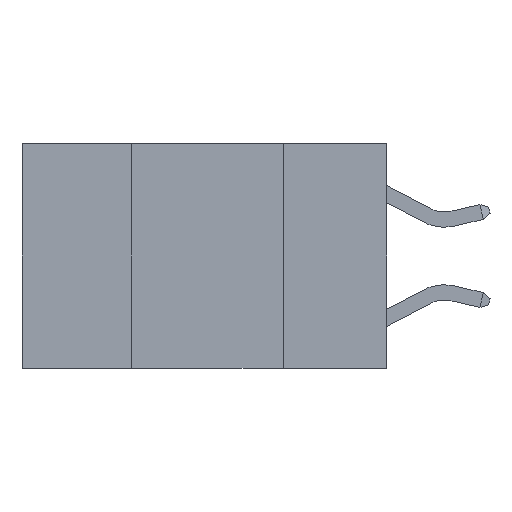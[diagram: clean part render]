
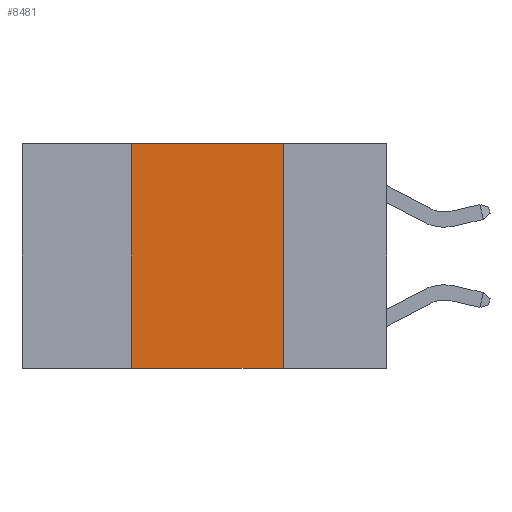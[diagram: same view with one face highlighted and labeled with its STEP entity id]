
A CAD part, left-side view. The second image highlights one B-rep face of the part: STEP entity #8481.
In plain terms, the highlighted planar face has unit normal (-1, 0, 0).
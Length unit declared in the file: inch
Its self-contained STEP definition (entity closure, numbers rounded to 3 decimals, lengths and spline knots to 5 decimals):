
#514 = DIRECTION ( 'NONE',  ( 0., -1., 0. ) ) ;
#793 = VERTEX_POINT ( 'NONE', #10084 ) ;
#930 = EDGE_CURVE ( 'NONE', #11056, #10215, #8560, .T. ) ;
#1129 = AXIS2_PLACEMENT_3D ( 'NONE', #6669, #11024, #2192 ) ;
#1268 = VECTOR ( 'NONE', #514, 39.37008 ) ;
#1642 = DIRECTION ( 'NONE',  ( 0., 0., -1. ) ) ;
#1764 = CARTESIAN_POINT ( 'NONE',  ( 0., 0.17, 0. ) ) ;
#1813 = EDGE_CURVE ( 'NONE', #6549, #793, #1833, .T. ) ;
#1833 = LINE ( 'NONE', #5180, #7843 ) ;
#2093 = CARTESIAN_POINT ( 'NONE',  ( 0., 0.42, -0.37 ) ) ;
#2192 = DIRECTION ( 'NONE',  ( 0., 0., -1. ) ) ;
#2552 = ORIENTED_EDGE ( 'NONE', *, *, #4462, .T. ) ;
#2690 = DIRECTION ( 'NONE',  ( 0., 0., 1. ) ) ;
#3554 = ORIENTED_EDGE ( 'NONE', *, *, #10961, .F. ) ;
#4025 = ORIENTED_EDGE ( 'NONE', *, *, #1813, .F. ) ;
#4067 = CARTESIAN_POINT ( 'NONE',  ( 0., 0.6, -0.37 ) ) ;
#4462 = EDGE_CURVE ( 'NONE', #6549, #10215, #10978, .T. ) ;
#5174 = CARTESIAN_POINT ( 'NONE',  ( 0., 0.17, 0. ) ) ;
#5180 = CARTESIAN_POINT ( 'NONE',  ( 0., 0.42, 0. ) ) ;
#5622 = CARTESIAN_POINT ( 'NONE',  ( 0., 0.6, 0. ) ) ;
#5777 = ORIENTED_EDGE ( 'NONE', *, *, #930, .F. ) ;
#6487 = LINE ( 'NONE', #5622, #1268 ) ;
#6549 = VERTEX_POINT ( 'NONE', #2093 ) ;
#6641 = CARTESIAN_POINT ( 'NONE',  ( 0., 0.17, -0.37 ) ) ;
#6669 = CARTESIAN_POINT ( 'NONE',  ( 0., 0.6, 0. ) ) ;
#7843 = VECTOR ( 'NONE', #2690, 39.37008 ) ;
#8167 = EDGE_LOOP ( 'NONE', ( #5777, #3554, #4025, #2552 ) ) ;
#8424 = FACE_OUTER_BOUND ( 'NONE', #8167, .T. ) ;
#8481 = ADVANCED_FACE ( 'NONE', ( #8424 ), #10054, .F. ) ;
#8484 = DIRECTION ( 'NONE',  ( 0., -1., 0. ) ) ;
#8560 = LINE ( 'NONE', #1764, #10034 ) ;
#10034 = VECTOR ( 'NONE', #1642, 39.37008 ) ;
#10054 = PLANE ( 'NONE',  #1129 ) ;
#10084 = CARTESIAN_POINT ( 'NONE',  ( 0., 0.42, 0. ) ) ;
#10215 = VERTEX_POINT ( 'NONE', #6641 ) ;
#10371 = VECTOR ( 'NONE', #8484, 39.37008 ) ;
#10961 = EDGE_CURVE ( 'NONE', #793, #11056, #6487, .T. ) ;
#10978 = LINE ( 'NONE', #4067, #10371 ) ;
#11024 = DIRECTION ( 'NONE',  ( 1., 0., 0. ) ) ;
#11056 = VERTEX_POINT ( 'NONE', #5174 ) ;
